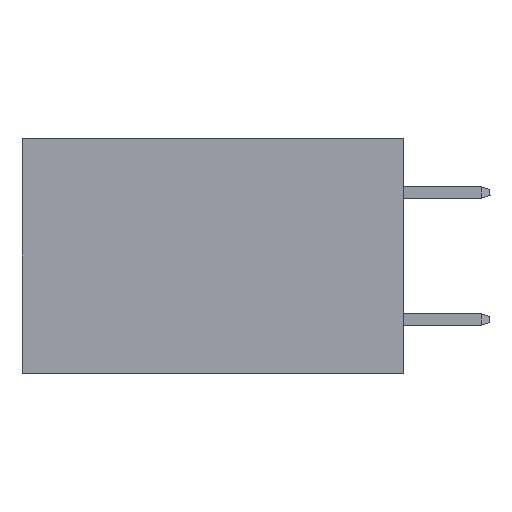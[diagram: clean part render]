
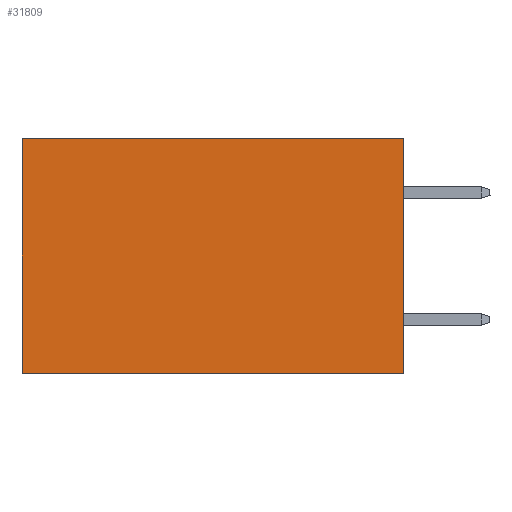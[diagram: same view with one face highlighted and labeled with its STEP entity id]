
A CAD part, left-side view. The second image highlights one B-rep face of the part: STEP entity #31809.
In plain terms, the highlighted planar face has unit normal (-1, 0, 0).
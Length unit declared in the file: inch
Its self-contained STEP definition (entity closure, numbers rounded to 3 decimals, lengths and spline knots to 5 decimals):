
#2832 = LINE ( 'NONE', #14130, #13671 ) ;
#2883 = VECTOR ( 'NONE', #26933, 39.37008 ) ;
#3411 = CARTESIAN_POINT ( 'NONE',  ( 0.2875, 0., 0. ) ) ;
#3824 = PLANE ( 'NONE',  #26553 ) ;
#4098 = LINE ( 'NONE', #27131, #2883 ) ;
#4196 = DIRECTION ( 'NONE',  ( 0., 0., -1. ) ) ;
#5529 = ORIENTED_EDGE ( 'NONE', *, *, #11179, .F. ) ;
#6378 = DIRECTION ( 'NONE',  ( 0., 0., -1. ) ) ;
#7258 = CARTESIAN_POINT ( 'NONE',  ( 0.2875, 0., -0.37 ) ) ;
#9307 = CARTESIAN_POINT ( 'NONE',  ( 0.2875, 0., 0. ) ) ;
#9426 = VERTEX_POINT ( 'NONE', #7258 ) ;
#9739 = DIRECTION ( 'NONE',  ( 0., 1., 0. ) ) ;
#10158 = ORIENTED_EDGE ( 'NONE', *, *, #35064, .T. ) ;
#11179 = EDGE_CURVE ( 'NONE', #9426, #21292, #12531, .T. ) ;
#11649 = EDGE_CURVE ( 'NONE', #17487, #9426, #26429, .T. ) ;
#12450 = CARTESIAN_POINT ( 'NONE',  ( 0.2875, 0.6, 0. ) ) ;
#12531 = LINE ( 'NONE', #35179, #31407 ) ;
#13466 = CARTESIAN_POINT ( 'NONE',  ( 0.2875, 0.6, -0.37 ) ) ;
#13671 = VECTOR ( 'NONE', #34206, 39.37008 ) ;
#14130 = CARTESIAN_POINT ( 'NONE',  ( 0.2875, 0.6, 0. ) ) ;
#14836 = VERTEX_POINT ( 'NONE', #12450 ) ;
#16561 = VECTOR ( 'NONE', #6378, 39.37008 ) ;
#17487 = VERTEX_POINT ( 'NONE', #9307 ) ;
#17921 = FACE_OUTER_BOUND ( 'NONE', #20149, .T. ) ;
#20149 = EDGE_LOOP ( 'NONE', ( #10158, #5529, #27347, #24606 ) ) ;
#20884 = CARTESIAN_POINT ( 'NONE',  ( 0.2875, 0., 0. ) ) ;
#21292 = VERTEX_POINT ( 'NONE', #13466 ) ;
#24606 = ORIENTED_EDGE ( 'NONE', *, *, #32189, .T. ) ;
#26429 = LINE ( 'NONE', #3411, #16561 ) ;
#26553 = AXIS2_PLACEMENT_3D ( 'NONE', #20884, #32228, #4196 ) ;
#26933 = DIRECTION ( 'NONE',  ( 0., 1., 0. ) ) ;
#27131 = CARTESIAN_POINT ( 'NONE',  ( 0.2875, 0., 0. ) ) ;
#27347 = ORIENTED_EDGE ( 'NONE', *, *, #11649, .F. ) ;
#31407 = VECTOR ( 'NONE', #9739, 39.37008 ) ;
#31809 = ADVANCED_FACE ( 'NONE', ( #17921 ), #3824, .F. ) ;
#32189 = EDGE_CURVE ( 'NONE', #17487, #14836, #4098, .T. ) ;
#32228 = DIRECTION ( 'NONE',  ( 1., 0., 0. ) ) ;
#34206 = DIRECTION ( 'NONE',  ( 0., 0., -1. ) ) ;
#35064 = EDGE_CURVE ( 'NONE', #14836, #21292, #2832, .T. ) ;
#35179 = CARTESIAN_POINT ( 'NONE',  ( 0.2875, 0., -0.37 ) ) ;
